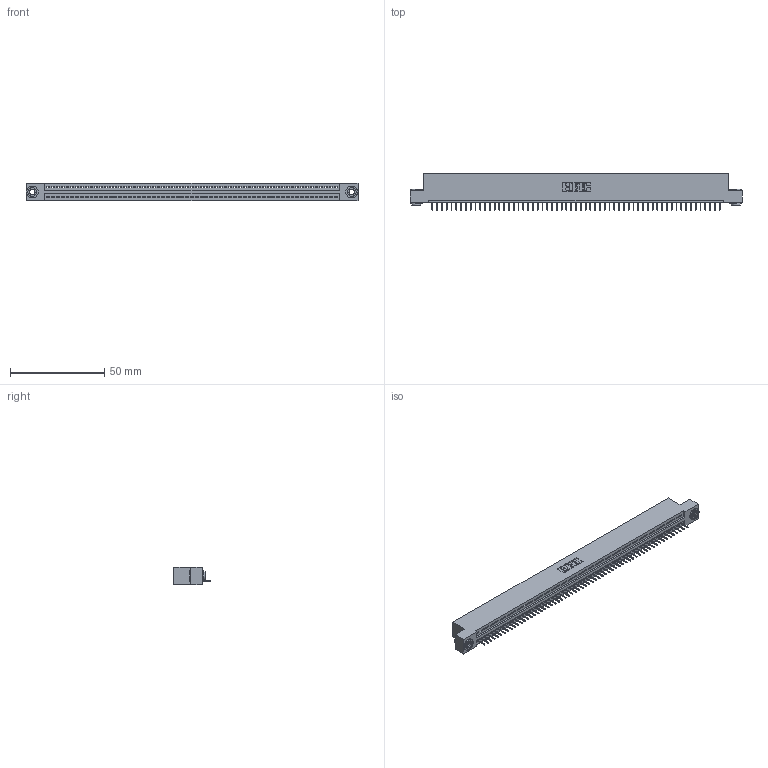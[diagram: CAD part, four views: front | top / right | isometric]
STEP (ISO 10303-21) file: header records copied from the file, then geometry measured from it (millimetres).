
FILE_DESCRIPTION (( 'STEP AP203' ), '1' );
FILE_NAME ('395-061-524-103.STEP', '2018-11-23T21:24:07', ( '' ), ( '' ), 'SwSTEP 2.0', 'SolidWorks 2016', '' );
FILE_SCHEMA (( 'CONFIG_CONTROL_DESIGN' ));
Length unit declared in the file: inch
Products named in the file (4): 345-292-001_345-293-124; 395-061-524-103; 345-250-002_345-250-002-102; 345 Part_Flush Mounting Lugs - 0.156 Dia-TH
Assembly tree (64 placements, depth 2):
  395-061-524-103
    345 Part_Flush Mounting Lugs - 0.156 Dia-TH
    345-292-001_345-293-124  x61
    345-250-002_345-250-002-102  x2
Bounding box: 176.15 x 19.35 x 9.4 mm (x, y, z)
Volume: 16664.9 mm3; surface area: 21848.4 mm2
Topology: 64 solids, 64 shells, 3946 faces, 11397 edges, 7350 vertices
Faces by surface type: plane 2896, cylinder 1042, cone 8
Entity records: 44076 total; most frequent: CARTESIAN_POINT 7610, ORIENTED_EDGE 7598, DIRECTION 6651, EDGE_CURVE 3799, LINE 3403, VECTOR 3403, VERTEX_POINT 2526, AXIS2_PLACEMENT_3D 1624
